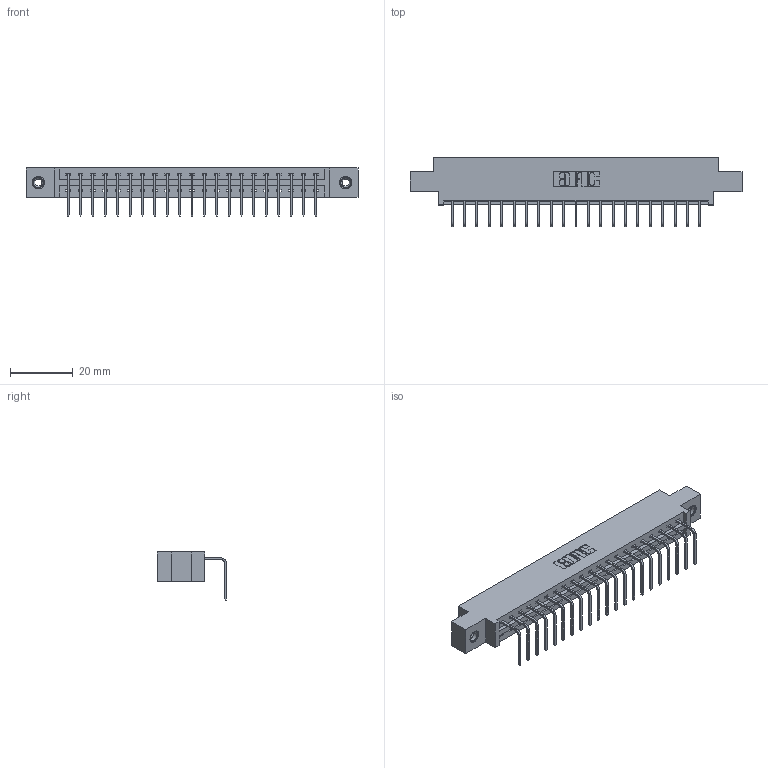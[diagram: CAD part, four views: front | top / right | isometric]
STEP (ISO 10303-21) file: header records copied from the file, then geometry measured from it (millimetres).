
FILE_DESCRIPTION (( 'STEP AP203' ), '1' );
FILE_NAME ('337-021-558-608.STEP', '2018-08-05T12:11:58', ( '' ), ( '' ), 'SwSTEP 2.0', 'SolidWorks 2016', '' );
FILE_SCHEMA (( 'CONFIG_CONTROL_DESIGN' ));
Length unit declared in the file: inch
Products named in the file (4): 337 Part_0.170 Offset - 0.156 Dia-TI; 345-292-001_558 Tail - 2; 345-250-001_345-250-003-102; 337-021-558-608
Assembly tree (24 placements, depth 2):
  337-021-558-608
    337 Part_0.170 Offset - 0.156 Dia-TI
    345-292-001_558 Tail - 2  x21
    345-250-001_345-250-003-102  x2
Bounding box: 106.22 x 22.17 x 15.37 mm (x, y, z)
Volume: 10723.2 mm3; surface area: 11520.3 mm2
Topology: 24 solids, 24 shells, 1522 faces, 4533 edges, 2986 vertices
Faces by surface type: plane 1114, cylinder 392, cone 12, torus 4
Entity records: 19728 total; most frequent: CARTESIAN_POINT 3416, ORIENTED_EDGE 3366, DIRECTION 2951, EDGE_CURVE 1683, LINE 1535, VECTOR 1535, VERTEX_POINT 1116, AXIS2_PLACEMENT_3D 708
